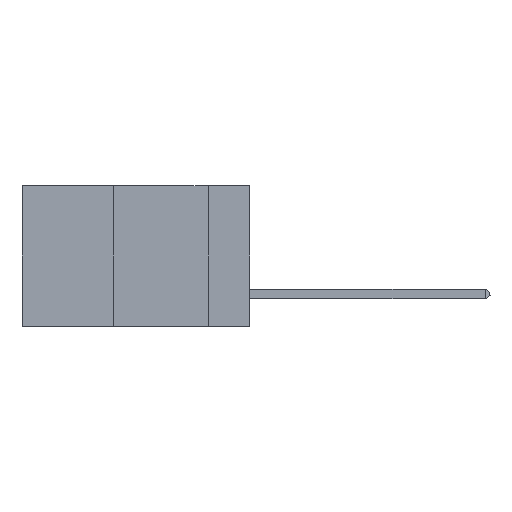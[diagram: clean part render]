
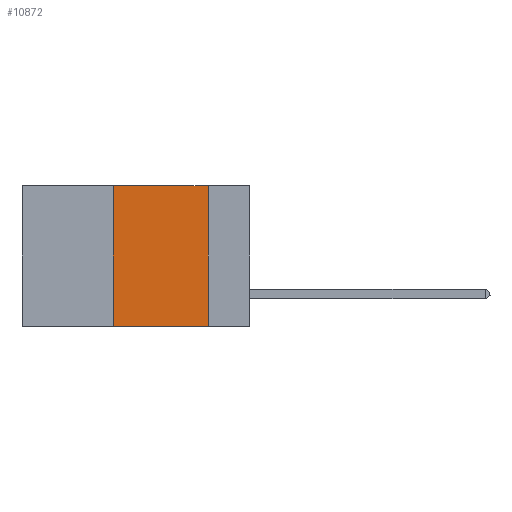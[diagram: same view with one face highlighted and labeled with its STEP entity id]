
A CAD part, left-side view. The second image highlights one B-rep face of the part: STEP entity #10872.
In plain terms, the highlighted planar face has unit normal (-1, 0, 0).
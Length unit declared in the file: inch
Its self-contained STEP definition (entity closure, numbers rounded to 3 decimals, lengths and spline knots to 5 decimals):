
#28 = CARTESIAN_POINT ( 'NONE',  ( 0., 0.11, 0. ) ) ;
#455 = DIRECTION ( 'NONE',  ( 0., 0., 1. ) ) ;
#474 = CARTESIAN_POINT ( 'NONE',  ( 0., 0.11, -0.37 ) ) ;
#1019 = LINE ( 'NONE', #17199, #13221 ) ;
#1170 = EDGE_CURVE ( 'NONE', #20273, #20320, #14767, .T. ) ;
#1256 = CARTESIAN_POINT ( 'NONE',  ( 0., 0.6, -0.37 ) ) ;
#1955 = CARTESIAN_POINT ( 'NONE',  ( 0., 0.36, 0. ) ) ;
#3577 = CARTESIAN_POINT ( 'NONE',  ( 0., 0.36, -0.37 ) ) ;
#5533 = DIRECTION ( 'NONE',  ( 0., 0., -1. ) ) ;
#5658 = CARTESIAN_POINT ( 'NONE',  ( 0., 0.11, 0. ) ) ;
#5878 = DIRECTION ( 'NONE',  ( 0., -1., 0. ) ) ;
#6117 = DIRECTION ( 'NONE',  ( 1., 0., 0. ) ) ;
#6901 = EDGE_CURVE ( 'NONE', #13670, #20320, #13627, .T. ) ;
#8133 = AXIS2_PLACEMENT_3D ( 'NONE', #18956, #6117, #12583 ) ;
#10150 = DIRECTION ( 'NONE',  ( 0., -1., 0. ) ) ;
#10872 = ADVANCED_FACE ( 'NONE', ( #20321 ), #11000, .F. ) ;
#11000 = PLANE ( 'NONE',  #8133 ) ;
#11218 = ORIENTED_EDGE ( 'NONE', *, *, #15693, .F. ) ;
#12583 = DIRECTION ( 'NONE',  ( 0., 0., -1. ) ) ;
#13221 = VECTOR ( 'NONE', #455, 39.37008 ) ;
#13270 = ORIENTED_EDGE ( 'NONE', *, *, #14739, .F. ) ;
#13514 = VECTOR ( 'NONE', #10150, 39.37008 ) ;
#13563 = VECTOR ( 'NONE', #5533, 39.37008 ) ;
#13627 = LINE ( 'NONE', #1256, #14840 ) ;
#13670 = VERTEX_POINT ( 'NONE', #3577 ) ;
#14739 = EDGE_CURVE ( 'NONE', #18797, #20273, #17705, .T. ) ;
#14767 = LINE ( 'NONE', #5658, #13563 ) ;
#14840 = VECTOR ( 'NONE', #5878, 39.37008 ) ;
#15693 = EDGE_CURVE ( 'NONE', #13670, #18797, #1019, .T. ) ;
#15909 = ORIENTED_EDGE ( 'NONE', *, *, #1170, .F. ) ;
#16332 = CARTESIAN_POINT ( 'NONE',  ( 0., 0.6, 0. ) ) ;
#17199 = CARTESIAN_POINT ( 'NONE',  ( 0., 0.36, 0. ) ) ;
#17705 = LINE ( 'NONE', #16332, #13514 ) ;
#17920 = EDGE_LOOP ( 'NONE', ( #15909, #13270, #11218, #18288 ) ) ;
#18288 = ORIENTED_EDGE ( 'NONE', *, *, #6901, .T. ) ;
#18797 = VERTEX_POINT ( 'NONE', #1955 ) ;
#18956 = CARTESIAN_POINT ( 'NONE',  ( 0., 0.6, 0. ) ) ;
#20273 = VERTEX_POINT ( 'NONE', #28 ) ;
#20320 = VERTEX_POINT ( 'NONE', #474 ) ;
#20321 = FACE_OUTER_BOUND ( 'NONE', #17920, .T. ) ;
